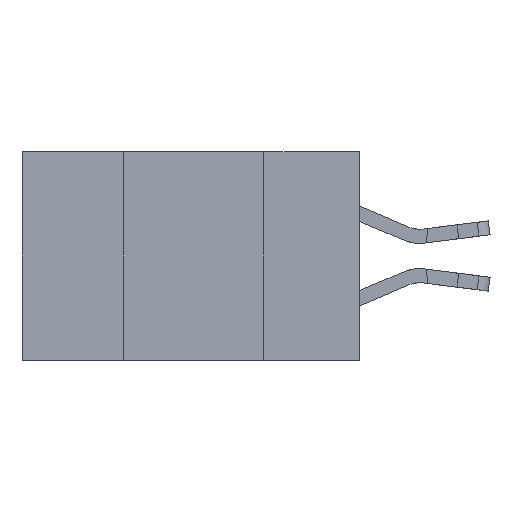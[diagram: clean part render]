
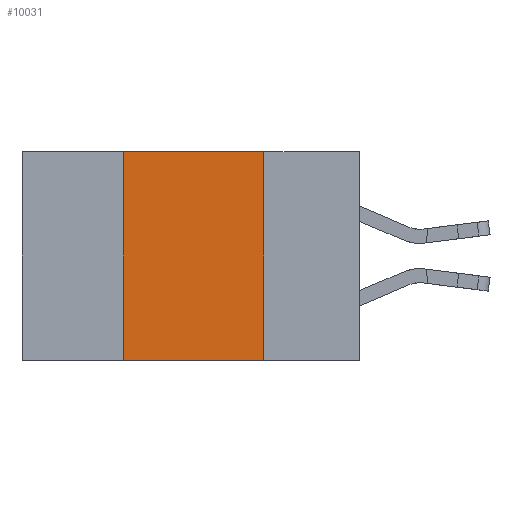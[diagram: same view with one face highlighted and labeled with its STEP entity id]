
A CAD part, left-side view. The second image highlights one B-rep face of the part: STEP entity #10031.
In plain terms, the highlighted planar face has unit normal (-1, 0, 0).
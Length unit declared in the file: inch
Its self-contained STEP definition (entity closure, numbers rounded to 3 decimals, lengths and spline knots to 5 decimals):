
#103 = ORIENTED_EDGE ( 'NONE', *, *, #16351, .F. ) ;
#847 = LINE ( 'NONE', #19647, #20945 ) ;
#925 = AXIS2_PLACEMENT_3D ( 'NONE', #7750, #9083, #18958 ) ;
#1192 = EDGE_LOOP ( 'NONE', ( #103, #3205, #20956, #14082 ) ) ;
#1720 = DIRECTION ( 'NONE',  ( 0., 0., 1. ) ) ;
#2178 = DIRECTION ( 'NONE',  ( 0., -1., 0. ) ) ;
#2250 = LINE ( 'NONE', #16003, #14714 ) ;
#3205 = ORIENTED_EDGE ( 'NONE', *, *, #9514, .F. ) ;
#3473 = FACE_OUTER_BOUND ( 'NONE', #1192, .T. ) ;
#3761 = CARTESIAN_POINT ( 'NONE',  ( 0., 0.6, -0.37 ) ) ;
#4788 = VERTEX_POINT ( 'NONE', #20594 ) ;
#6067 = LINE ( 'NONE', #13363, #11088 ) ;
#7548 = EDGE_CURVE ( 'NONE', #17252, #4788, #847, .T. ) ;
#7750 = CARTESIAN_POINT ( 'NONE',  ( 0., 0.6, 0. ) ) ;
#8207 = EDGE_CURVE ( 'NONE', #17252, #20969, #19632, .T. ) ;
#8651 = CARTESIAN_POINT ( 'NONE',  ( 0., 0.42, -0.37 ) ) ;
#9083 = DIRECTION ( 'NONE',  ( 1., 0., 0. ) ) ;
#9514 = EDGE_CURVE ( 'NONE', #4788, #14993, #6067, .T. ) ;
#9903 = CARTESIAN_POINT ( 'NONE',  ( 0., 0.17, 0. ) ) ;
#10031 = ADVANCED_FACE ( 'NONE', ( #3473 ), #18827, .F. ) ;
#10223 = CARTESIAN_POINT ( 'NONE',  ( 0., 0.17, -0.37 ) ) ;
#11088 = VECTOR ( 'NONE', #14956, 39.37008 ) ;
#12220 = VECTOR ( 'NONE', #2178, 39.37008 ) ;
#13363 = CARTESIAN_POINT ( 'NONE',  ( 0., 0.6, 0. ) ) ;
#14082 = ORIENTED_EDGE ( 'NONE', *, *, #8207, .T. ) ;
#14714 = VECTOR ( 'NONE', #17780, 39.37008 ) ;
#14956 = DIRECTION ( 'NONE',  ( 0., -1., 0. ) ) ;
#14993 = VERTEX_POINT ( 'NONE', #9903 ) ;
#16003 = CARTESIAN_POINT ( 'NONE',  ( 0., 0.17, 0. ) ) ;
#16351 = EDGE_CURVE ( 'NONE', #14993, #20969, #2250, .T. ) ;
#17252 = VERTEX_POINT ( 'NONE', #8651 ) ;
#17780 = DIRECTION ( 'NONE',  ( 0., 0., -1. ) ) ;
#18827 = PLANE ( 'NONE',  #925 ) ;
#18958 = DIRECTION ( 'NONE',  ( 0., 0., -1. ) ) ;
#19632 = LINE ( 'NONE', #3761, #12220 ) ;
#19647 = CARTESIAN_POINT ( 'NONE',  ( 0., 0.42, 0. ) ) ;
#20594 = CARTESIAN_POINT ( 'NONE',  ( 0., 0.42, 0. ) ) ;
#20945 = VECTOR ( 'NONE', #1720, 39.37008 ) ;
#20956 = ORIENTED_EDGE ( 'NONE', *, *, #7548, .F. ) ;
#20969 = VERTEX_POINT ( 'NONE', #10223 ) ;
